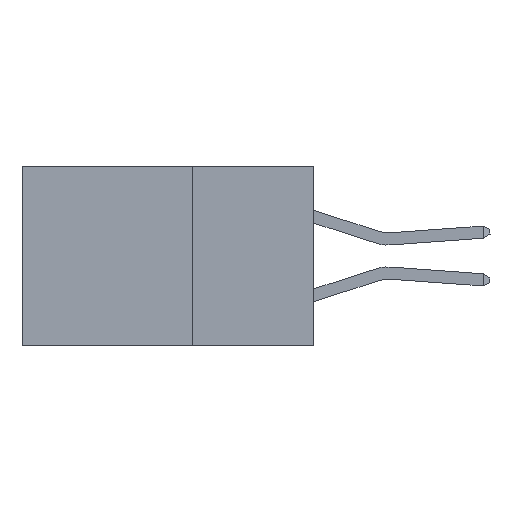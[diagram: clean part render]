
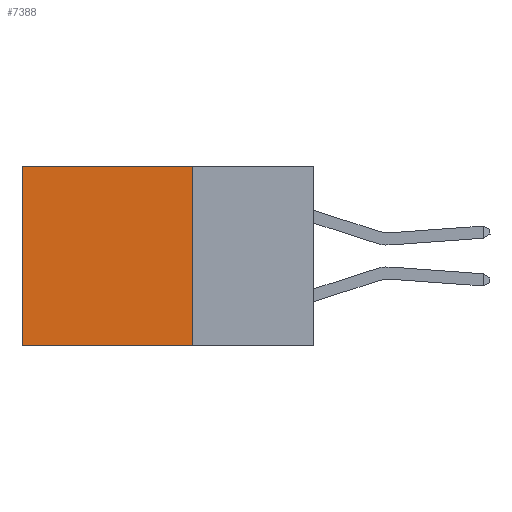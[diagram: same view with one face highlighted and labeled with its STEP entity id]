
A CAD part, left-side view. The second image highlights one B-rep face of the part: STEP entity #7388.
In plain terms, the highlighted planar face has unit normal (-1, 0, 0).
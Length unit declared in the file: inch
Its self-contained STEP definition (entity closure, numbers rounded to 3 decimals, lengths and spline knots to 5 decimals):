
#54 = DIRECTION ( 'NONE',  ( 1., 0., 0. ) ) ;
#827 = FACE_OUTER_BOUND ( 'NONE', #8400, .T. ) ;
#830 = VERTEX_POINT ( 'NONE', #7523 ) ;
#1642 = EDGE_CURVE ( 'NONE', #5327, #6036, #3473, .T. ) ;
#1683 = DIRECTION ( 'NONE',  ( 0., 0., -1. ) ) ;
#2709 = CARTESIAN_POINT ( 'NONE',  ( 0.2875, 0.25, 0. ) ) ;
#3348 = ORIENTED_EDGE ( 'NONE', *, *, #1642, .F. ) ;
#3473 = LINE ( 'NONE', #7075, #8170 ) ;
#3592 = EDGE_CURVE ( 'NONE', #830, #7053, #8222, .T. ) ;
#3732 = LINE ( 'NONE', #7571, #11882 ) ;
#4088 = AXIS2_PLACEMENT_3D ( 'NONE', #2709, #54, #1683 ) ;
#4770 = DIRECTION ( 'NONE',  ( 0., 0., -1. ) ) ;
#5327 = VERTEX_POINT ( 'NONE', #8523 ) ;
#6036 = VERTEX_POINT ( 'NONE', #10980 ) ;
#6153 = EDGE_CURVE ( 'NONE', #830, #5327, #3732, .T. ) ;
#6191 = DIRECTION ( 'NONE',  ( 0., 0., -1. ) ) ;
#6194 = ORIENTED_EDGE ( 'NONE', *, *, #6153, .F. ) ;
#7053 = VERTEX_POINT ( 'NONE', #11483 ) ;
#7075 = CARTESIAN_POINT ( 'NONE',  ( 0.2875, 0.25, -0.37 ) ) ;
#7388 = ADVANCED_FACE ( 'NONE', ( #827 ), #10982, .F. ) ;
#7523 = CARTESIAN_POINT ( 'NONE',  ( 0.2875, 0.25, 0. ) ) ;
#7571 = CARTESIAN_POINT ( 'NONE',  ( 0.2875, 0.25, 0. ) ) ;
#8170 = VECTOR ( 'NONE', #10785, 39.37008 ) ;
#8222 = LINE ( 'NONE', #9127, #9303 ) ;
#8400 = EDGE_LOOP ( 'NONE', ( #9029, #3348, #6194, #10451 ) ) ;
#8523 = CARTESIAN_POINT ( 'NONE',  ( 0.2875, 0.25, -0.37 ) ) ;
#8805 = VECTOR ( 'NONE', #6191, 39.37008 ) ;
#9029 = ORIENTED_EDGE ( 'NONE', *, *, #10190, .T. ) ;
#9127 = CARTESIAN_POINT ( 'NONE',  ( 0.2875, 0.25, 0. ) ) ;
#9303 = VECTOR ( 'NONE', #10951, 39.37008 ) ;
#9790 = LINE ( 'NONE', #10647, #8805 ) ;
#10190 = EDGE_CURVE ( 'NONE', #7053, #6036, #9790, .T. ) ;
#10451 = ORIENTED_EDGE ( 'NONE', *, *, #3592, .T. ) ;
#10647 = CARTESIAN_POINT ( 'NONE',  ( 0.2875, 0.6, 0. ) ) ;
#10785 = DIRECTION ( 'NONE',  ( 0., 1., 0. ) ) ;
#10951 = DIRECTION ( 'NONE',  ( 0., 1., 0. ) ) ;
#10980 = CARTESIAN_POINT ( 'NONE',  ( 0.2875, 0.6, -0.37 ) ) ;
#10982 = PLANE ( 'NONE',  #4088 ) ;
#11483 = CARTESIAN_POINT ( 'NONE',  ( 0.2875, 0.6, 0. ) ) ;
#11882 = VECTOR ( 'NONE', #4770, 39.37008 ) ;
